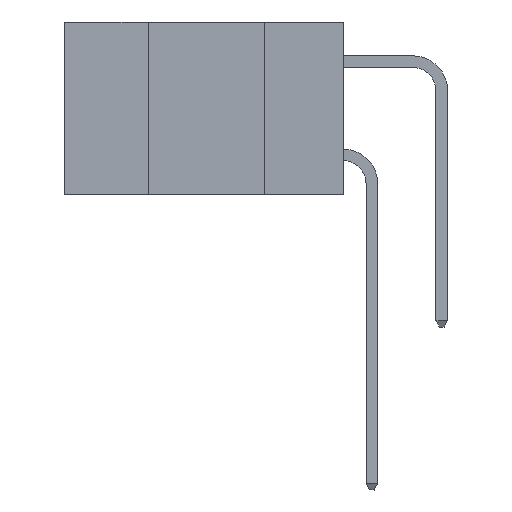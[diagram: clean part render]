
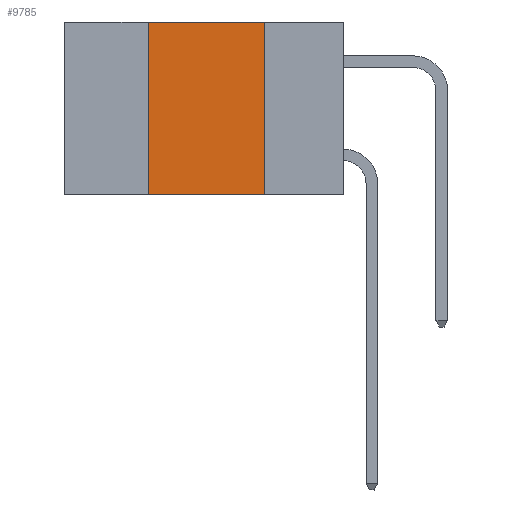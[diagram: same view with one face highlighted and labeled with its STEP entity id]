
A CAD part, left-side view. The second image highlights one B-rep face of the part: STEP entity #9785.
In plain terms, the highlighted planar face has unit normal (-1, 0, 0).
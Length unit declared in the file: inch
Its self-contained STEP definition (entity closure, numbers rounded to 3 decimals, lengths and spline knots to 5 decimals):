
#68 = DIRECTION ( 'NONE',  ( 0., 0., -1. ) ) ;
#135 = EDGE_CURVE ( 'NONE', #9555, #13143, #12666, .T. ) ;
#424 = VECTOR ( 'NONE', #10474, 39.37008 ) ;
#510 = VECTOR ( 'NONE', #68, 39.37008 ) ;
#2044 = LINE ( 'NONE', #6236, #424 ) ;
#2200 = DIRECTION ( 'NONE',  ( 0., -1., 0. ) ) ;
#2693 = VERTEX_POINT ( 'NONE', #10360 ) ;
#2898 = EDGE_CURVE ( 'NONE', #12597, #13143, #5561, .T. ) ;
#2996 = ORIENTED_EDGE ( 'NONE', *, *, #5079, .F. ) ;
#3001 = CARTESIAN_POINT ( 'NONE',  ( 0., 0.17, 0. ) ) ;
#3350 = LINE ( 'NONE', #11785, #4629 ) ;
#3780 = ORIENTED_EDGE ( 'NONE', *, *, #2898, .T. ) ;
#4066 = FACE_OUTER_BOUND ( 'NONE', #12107, .T. ) ;
#4629 = VECTOR ( 'NONE', #10741, 39.37008 ) ;
#4891 = CARTESIAN_POINT ( 'NONE',  ( 0., 0.6, 0. ) ) ;
#5079 = EDGE_CURVE ( 'NONE', #12597, #2693, #2044, .T. ) ;
#5561 = LINE ( 'NONE', #8636, #13103 ) ;
#6236 = CARTESIAN_POINT ( 'NONE',  ( 0., 0.42, -0.37 ) ) ;
#6300 = CARTESIAN_POINT ( 'NONE',  ( 0., 0.42, -0.37 ) ) ;
#7040 = PLANE ( 'NONE',  #11607 ) ;
#8227 = ORIENTED_EDGE ( 'NONE', *, *, #135, .F. ) ;
#8289 = EDGE_CURVE ( 'NONE', #2693, #9555, #3350, .T. ) ;
#8636 = CARTESIAN_POINT ( 'NONE',  ( 0., 0.6, -0.37 ) ) ;
#9118 = DIRECTION ( 'NONE',  ( 1., 0., 0. ) ) ;
#9380 = CARTESIAN_POINT ( 'NONE',  ( 0., 0.17, -0.37 ) ) ;
#9555 = VERTEX_POINT ( 'NONE', #3001 ) ;
#9785 = ADVANCED_FACE ( 'NONE', ( #4066 ), #7040, .F. ) ;
#10360 = CARTESIAN_POINT ( 'NONE',  ( 0., 0.42, 0. ) ) ;
#10474 = DIRECTION ( 'NONE',  ( 0., 0., 1. ) ) ;
#10741 = DIRECTION ( 'NONE',  ( 0., -1., 0. ) ) ;
#10748 = ORIENTED_EDGE ( 'NONE', *, *, #8289, .F. ) ;
#11201 = CARTESIAN_POINT ( 'NONE',  ( 0., 0.17, -0.37 ) ) ;
#11607 = AXIS2_PLACEMENT_3D ( 'NONE', #4891, #9118, #12318 ) ;
#11785 = CARTESIAN_POINT ( 'NONE',  ( 0., 0.6, 0. ) ) ;
#12107 = EDGE_LOOP ( 'NONE', ( #8227, #10748, #2996, #3780 ) ) ;
#12318 = DIRECTION ( 'NONE',  ( 0., 0., -1. ) ) ;
#12597 = VERTEX_POINT ( 'NONE', #6300 ) ;
#12666 = LINE ( 'NONE', #9380, #510 ) ;
#13103 = VECTOR ( 'NONE', #2200, 39.37008 ) ;
#13143 = VERTEX_POINT ( 'NONE', #11201 ) ;
